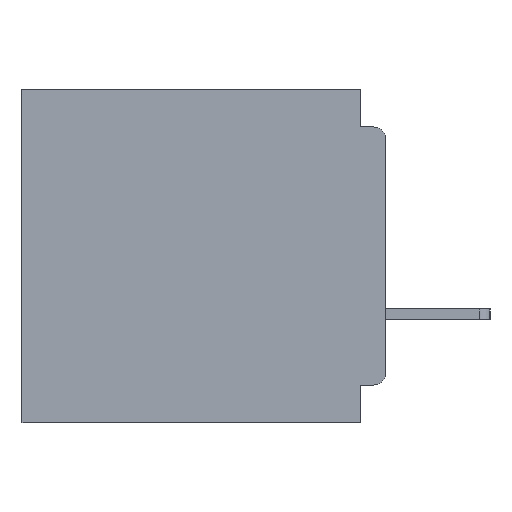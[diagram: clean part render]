
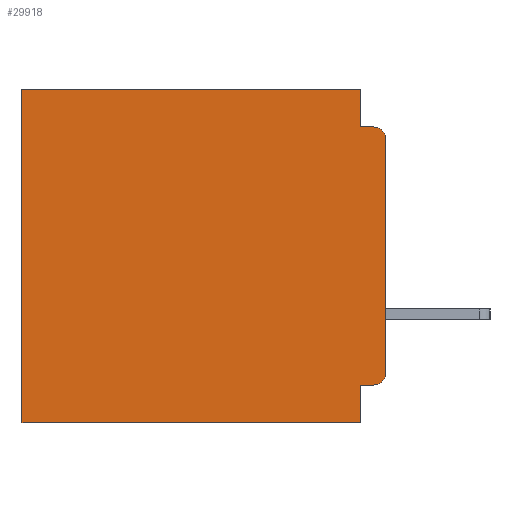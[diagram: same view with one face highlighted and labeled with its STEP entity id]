
A CAD part, left-side view. The second image highlights one B-rep face of the part: STEP entity #29918.
In plain terms, the highlighted planar face has unit normal (-1, 0, 0).
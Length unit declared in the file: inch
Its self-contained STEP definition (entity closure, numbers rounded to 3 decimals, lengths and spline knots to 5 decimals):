
#1440 = ORIENTED_EDGE ( 'NONE', *, *, #25565, .T. ) ;
#1461 = DIRECTION ( 'NONE',  ( 0., 1., 0. ) ) ;
#2223 = EDGE_CURVE ( 'NONE', #3148, #29399, #16054, .T. ) ;
#2430 = CARTESIAN_POINT ( 'NONE',  ( 0.3, 0.015, -0.355 ) ) ;
#2770 = LINE ( 'NONE', #38667, #12456 ) ;
#3148 = VERTEX_POINT ( 'NONE', #28192 ) ;
#3982 = CARTESIAN_POINT ( 'NONE',  ( 0.3, 0.031, -0.045 ) ) ;
#4273 = CARTESIAN_POINT ( 'NONE',  ( 0.3, 0.015, -0.06 ) ) ;
#6586 = DIRECTION ( 'NONE',  ( -1., 0., 0. ) ) ;
#7117 = LINE ( 'NONE', #18257, #24035 ) ;
#7125 = LINE ( 'NONE', #17382, #39488 ) ;
#7506 = VERTEX_POINT ( 'NONE', #3982 ) ;
#7515 = EDGE_CURVE ( 'NONE', #16776, #40612, #2770, .T. ) ;
#7533 = CARTESIAN_POINT ( 'NONE',  ( 0.3, 0.015, -0.045 ) ) ;
#7589 = DIRECTION ( 'NONE',  ( 0., 0., -1. ) ) ;
#8508 = VERTEX_POINT ( 'NONE', #15985 ) ;
#10014 = CARTESIAN_POINT ( 'NONE',  ( 0.3, 0., -0.4 ) ) ;
#11042 = CARTESIAN_POINT ( 'NONE',  ( 0.3, 0.031, -0.355 ) ) ;
#11453 = AXIS2_PLACEMENT_3D ( 'NONE', #10014, #13261, #35075 ) ;
#12456 = VECTOR ( 'NONE', #23290, 39.37008 ) ;
#12690 = LINE ( 'NONE', #15577, #29357 ) ;
#13261 = DIRECTION ( 'NONE',  ( 1., 0., 0. ) ) ;
#13490 = VERTEX_POINT ( 'NONE', #7533 ) ;
#14814 = CARTESIAN_POINT ( 'NONE',  ( 0.3, 0.031, -0.4 ) ) ;
#15577 = CARTESIAN_POINT ( 'NONE',  ( 0.3, 0., -0.4 ) ) ;
#15985 = CARTESIAN_POINT ( 'NONE',  ( 0.3, 0.437, 0. ) ) ;
#16054 = LINE ( 'NONE', #38400, #39809 ) ;
#16776 = VERTEX_POINT ( 'NONE', #2430 ) ;
#16839 = DIRECTION ( 'NONE',  ( 0., 0., -1. ) ) ;
#17382 = CARTESIAN_POINT ( 'NONE',  ( 0.3, 0.031, -0.4 ) ) ;
#17743 = EDGE_CURVE ( 'NONE', #40612, #17871, #7125, .T. ) ;
#17871 = VERTEX_POINT ( 'NONE', #14814 ) ;
#18257 = CARTESIAN_POINT ( 'NONE',  ( 0.3, 0., -0.045 ) ) ;
#19096 = VECTOR ( 'NONE', #16839, 39.37008 ) ;
#19959 = ORIENTED_EDGE ( 'NONE', *, *, #17743, .F. ) ;
#20055 = ORIENTED_EDGE ( 'NONE', *, *, #7515, .F. ) ;
#21396 = EDGE_CURVE ( 'NONE', #17871, #22141, #12690, .T. ) ;
#22025 = ORIENTED_EDGE ( 'NONE', *, *, #29152, .F. ) ;
#22141 = VERTEX_POINT ( 'NONE', #35071 ) ;
#22771 = EDGE_CURVE ( 'NONE', #16776, #29399, #38878, .T. ) ;
#23156 = LINE ( 'NONE', #39245, #36687 ) ;
#23290 = DIRECTION ( 'NONE',  ( 0., 1., 0. ) ) ;
#24035 = VECTOR ( 'NONE', #33669, 39.37008 ) ;
#24839 = ORIENTED_EDGE ( 'NONE', *, *, #22771, .T. ) ;
#24860 = DIRECTION ( 'NONE',  ( 0., 1., 0. ) ) ;
#25227 = DIRECTION ( 'NONE',  ( 0., 0., -1. ) ) ;
#25565 = EDGE_CURVE ( 'NONE', #3148, #13490, #36858, .T. ) ;
#25569 = CARTESIAN_POINT ( 'NONE',  ( 0.3, 0.015, -0.34 ) ) ;
#26280 = AXIS2_PLACEMENT_3D ( 'NONE', #25569, #6586, #28692 ) ;
#26327 = LINE ( 'NONE', #35382, #19096 ) ;
#26540 = DIRECTION ( 'NONE',  ( -1., 0., 0. ) ) ;
#26711 = DIRECTION ( 'NONE',  ( 0., 0., -1. ) ) ;
#28192 = CARTESIAN_POINT ( 'NONE',  ( 0.3, 0., -0.06 ) ) ;
#28692 = DIRECTION ( 'NONE',  ( 0., 0., -1. ) ) ;
#28849 = ORIENTED_EDGE ( 'NONE', *, *, #40474, .T. ) ;
#28858 = PLANE ( 'NONE',  #11453 ) ;
#28955 = AXIS2_PLACEMENT_3D ( 'NONE', #4273, #26540, #7589 ) ;
#29152 = EDGE_CURVE ( 'NONE', #7506, #13490, #7117, .T. ) ;
#29357 = VECTOR ( 'NONE', #24860, 39.37008 ) ;
#29399 = VERTEX_POINT ( 'NONE', #34973 ) ;
#29918 = ADVANCED_FACE ( 'NONE', ( #34116 ), #28858, .F. ) ;
#30956 = EDGE_LOOP ( 'NONE', ( #34950, #1440, #22025, #38116, #36873, #28849, #38215, #19959, #20055, #24839 ) ) ;
#31082 = LINE ( 'NONE', #40581, #38327 ) ;
#33131 = CARTESIAN_POINT ( 'NONE',  ( 0.3, 0.031, 0. ) ) ;
#33669 = DIRECTION ( 'NONE',  ( 0., -1., 0. ) ) ;
#34116 = FACE_OUTER_BOUND ( 'NONE', #30956, .T. ) ;
#34950 = ORIENTED_EDGE ( 'NONE', *, *, #2223, .F. ) ;
#34973 = CARTESIAN_POINT ( 'NONE',  ( 0.3, 0., -0.34 ) ) ;
#35069 = EDGE_CURVE ( 'NONE', #38869, #7506, #31082, .T. ) ;
#35071 = CARTESIAN_POINT ( 'NONE',  ( 0.3, 0.437, -0.4 ) ) ;
#35075 = DIRECTION ( 'NONE',  ( 0., 0., -1. ) ) ;
#35382 = CARTESIAN_POINT ( 'NONE',  ( 0.3, 0.437, -0.4 ) ) ;
#36687 = VECTOR ( 'NONE', #1461, 39.37008 ) ;
#36858 = CIRCLE ( 'NONE', #28955, 0.015 ) ;
#36873 = ORIENTED_EDGE ( 'NONE', *, *, #37779, .T. ) ;
#37779 = EDGE_CURVE ( 'NONE', #38869, #8508, #23156, .T. ) ;
#38116 = ORIENTED_EDGE ( 'NONE', *, *, #35069, .F. ) ;
#38215 = ORIENTED_EDGE ( 'NONE', *, *, #21396, .F. ) ;
#38327 = VECTOR ( 'NONE', #25227, 39.37008 ) ;
#38400 = CARTESIAN_POINT ( 'NONE',  ( 0.3, 0., -0.4 ) ) ;
#38491 = DIRECTION ( 'NONE',  ( 0., 0., -1. ) ) ;
#38667 = CARTESIAN_POINT ( 'NONE',  ( 0.3, 0., -0.355 ) ) ;
#38869 = VERTEX_POINT ( 'NONE', #33131 ) ;
#38878 = CIRCLE ( 'NONE', #26280, 0.015 ) ;
#39245 = CARTESIAN_POINT ( 'NONE',  ( 0.3, 0., 0. ) ) ;
#39488 = VECTOR ( 'NONE', #26711, 39.37008 ) ;
#39809 = VECTOR ( 'NONE', #38491, 39.37008 ) ;
#40474 = EDGE_CURVE ( 'NONE', #8508, #22141, #26327, .T. ) ;
#40581 = CARTESIAN_POINT ( 'NONE',  ( 0.3, 0.031, 0. ) ) ;
#40612 = VERTEX_POINT ( 'NONE', #11042 ) ;
